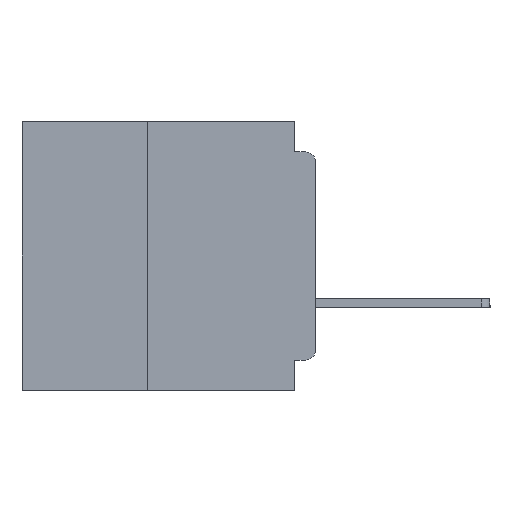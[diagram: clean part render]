
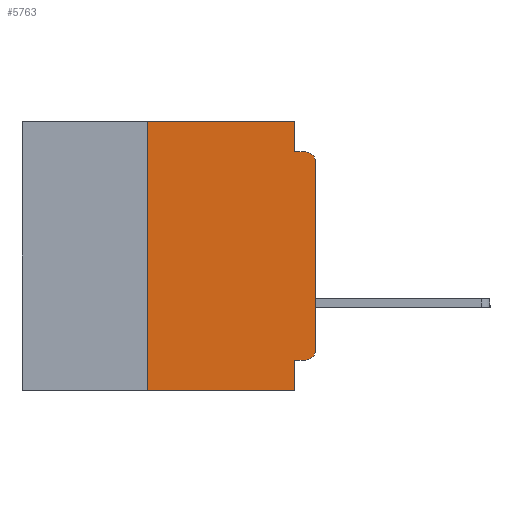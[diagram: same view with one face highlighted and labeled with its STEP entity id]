
A CAD part, left-side view. The second image highlights one B-rep face of the part: STEP entity #5763.
In plain terms, the highlighted planar face has unit normal (-1, 0, 0).
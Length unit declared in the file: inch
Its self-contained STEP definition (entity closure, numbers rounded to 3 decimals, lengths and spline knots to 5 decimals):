
#86 = CARTESIAN_POINT ( 'NONE',  ( 0., 0.437, -0.4 ) ) ;
#521 = EDGE_CURVE ( 'NONE', #8787, #3354, #33060, .T. ) ;
#1106 = ORIENTED_EDGE ( 'NONE', *, *, #25989, .T. ) ;
#1146 = EDGE_LOOP ( 'NONE', ( #22975, #1106, #11759, #16708, #17665, #4040, #8534, #8616, #25637, #13519 ) ) ;
#1576 = CARTESIAN_POINT ( 'NONE',  ( 0., 0.015, -0.06 ) ) ;
#1842 = VERTEX_POINT ( 'NONE', #36062 ) ;
#2887 = VECTOR ( 'NONE', #4983, 39.37008 ) ;
#2947 = CARTESIAN_POINT ( 'NONE',  ( 0., 0.031, 0. ) ) ;
#3354 = VERTEX_POINT ( 'NONE', #25470 ) ;
#3973 = EDGE_CURVE ( 'NONE', #3354, #33789, #15572, .T. ) ;
#4040 = ORIENTED_EDGE ( 'NONE', *, *, #521, .F. ) ;
#4382 = DIRECTION ( 'NONE',  ( 1., 0., 0. ) ) ;
#4648 = DIRECTION ( 'NONE',  ( 0., 0., -1. ) ) ;
#4983 = DIRECTION ( 'NONE',  ( 0., 0., 1. ) ) ;
#5763 = ADVANCED_FACE ( 'NONE', ( #27649 ), #25344, .F. ) ;
#5809 = LINE ( 'NONE', #11395, #28939 ) ;
#6555 = VECTOR ( 'NONE', #24130, 39.37008 ) ;
#7308 = AXIS2_PLACEMENT_3D ( 'NONE', #1576, #22741, #4648 ) ;
#8444 = LINE ( 'NONE', #30062, #6555 ) ;
#8534 = ORIENTED_EDGE ( 'NONE', *, *, #14722, .T. ) ;
#8616 = ORIENTED_EDGE ( 'NONE', *, *, #38856, .F. ) ;
#8787 = VERTEX_POINT ( 'NONE', #9365 ) ;
#9365 = CARTESIAN_POINT ( 'NONE',  ( 0., 0.25, -0.4 ) ) ;
#9541 = DIRECTION ( 'NONE',  ( 0., 0., -1. ) ) ;
#11395 = CARTESIAN_POINT ( 'NONE',  ( 0., 0., -0.045 ) ) ;
#11406 = CARTESIAN_POINT ( 'NONE',  ( 0., 0.015, -0.045 ) ) ;
#11514 = DIRECTION ( 'NONE',  ( 0., -1., 0. ) ) ;
#11759 = ORIENTED_EDGE ( 'NONE', *, *, #18655, .F. ) ;
#12653 = VERTEX_POINT ( 'NONE', #20048 ) ;
#13519 = ORIENTED_EDGE ( 'NONE', *, *, #16425, .T. ) ;
#13583 = DIRECTION ( 'NONE',  ( 0., -1., 0. ) ) ;
#14355 = CARTESIAN_POINT ( 'NONE',  ( 0., 0.031, -0.355 ) ) ;
#14722 = EDGE_CURVE ( 'NONE', #8787, #35647, #21296, .T. ) ;
#15084 = CIRCLE ( 'NONE', #7308, 0.015 ) ;
#15292 = CARTESIAN_POINT ( 'NONE',  ( 0., 0., -0.355 ) ) ;
#15412 = DIRECTION ( 'NONE',  ( 0., 1., 0. ) ) ;
#15527 = DIRECTION ( 'NONE',  ( -1., 0., 0. ) ) ;
#15572 = LINE ( 'NONE', #22582, #22631 ) ;
#15683 = CARTESIAN_POINT ( 'NONE',  ( 0., 0.031, -0.4 ) ) ;
#16425 = EDGE_CURVE ( 'NONE', #1842, #12653, #36123, .T. ) ;
#16708 = ORIENTED_EDGE ( 'NONE', *, *, #31094, .F. ) ;
#17665 = ORIENTED_EDGE ( 'NONE', *, *, #3973, .F. ) ;
#17697 = CARTESIAN_POINT ( 'NONE',  ( 0., 0., -0.06 ) ) ;
#18655 = EDGE_CURVE ( 'NONE', #25463, #28816, #5809, .T. ) ;
#20048 = CARTESIAN_POINT ( 'NONE',  ( 0., 0., -0.34 ) ) ;
#20964 = VECTOR ( 'NONE', #24192, 39.37008 ) ;
#21252 = DIRECTION ( 'NONE',  ( 0., -1., 0. ) ) ;
#21296 = LINE ( 'NONE', #86, #37208 ) ;
#22458 = CARTESIAN_POINT ( 'NONE',  ( 0., 0.437, 0. ) ) ;
#22582 = CARTESIAN_POINT ( 'NONE',  ( 0., 0.437, 0. ) ) ;
#22631 = VECTOR ( 'NONE', #13583, 39.37008 ) ;
#22741 = DIRECTION ( 'NONE',  ( -1., 0., 0. ) ) ;
#22803 = VERTEX_POINT ( 'NONE', #14355 ) ;
#22975 = ORIENTED_EDGE ( 'NONE', *, *, #28309, .T. ) ;
#23720 = AXIS2_PLACEMENT_3D ( 'NONE', #22458, #4382, #25475 ) ;
#24130 = DIRECTION ( 'NONE',  ( 0., 0., 1. ) ) ;
#24192 = DIRECTION ( 'NONE',  ( 0., 0., -1. ) ) ;
#25344 = PLANE ( 'NONE',  #23720 ) ;
#25463 = VERTEX_POINT ( 'NONE', #38220 ) ;
#25470 = CARTESIAN_POINT ( 'NONE',  ( 0., 0.25, 0. ) ) ;
#25475 = DIRECTION ( 'NONE',  ( 0., 0., -1. ) ) ;
#25637 = ORIENTED_EDGE ( 'NONE', *, *, #33869, .F. ) ;
#25989 = EDGE_CURVE ( 'NONE', #36343, #28816, #15084, .T. ) ;
#26809 = CARTESIAN_POINT ( 'NONE',  ( 0., 0.25, -0.4 ) ) ;
#27649 = FACE_OUTER_BOUND ( 'NONE', #1146, .T. ) ;
#28309 = EDGE_CURVE ( 'NONE', #12653, #36343, #8444, .T. ) ;
#28816 = VERTEX_POINT ( 'NONE', #11406 ) ;
#28939 = VECTOR ( 'NONE', #11514, 39.37008 ) ;
#28982 = LINE ( 'NONE', #2947, #20964 ) ;
#29943 = VECTOR ( 'NONE', #15412, 39.37008 ) ;
#30062 = CARTESIAN_POINT ( 'NONE',  ( 0., 0., 0. ) ) ;
#31094 = EDGE_CURVE ( 'NONE', #33789, #25463, #28982, .T. ) ;
#32571 = CARTESIAN_POINT ( 'NONE',  ( 0., 0.031, -0.4 ) ) ;
#33060 = LINE ( 'NONE', #26809, #2887 ) ;
#33516 = CARTESIAN_POINT ( 'NONE',  ( 0., 0.015, -0.34 ) ) ;
#33789 = VERTEX_POINT ( 'NONE', #38746 ) ;
#33869 = EDGE_CURVE ( 'NONE', #1842, #22803, #38789, .T. ) ;
#35641 = VECTOR ( 'NONE', #9541, 39.37008 ) ;
#35647 = VERTEX_POINT ( 'NONE', #32571 ) ;
#36062 = CARTESIAN_POINT ( 'NONE',  ( 0., 0.015, -0.355 ) ) ;
#36123 = CIRCLE ( 'NONE', #36284, 0.015 ) ;
#36284 = AXIS2_PLACEMENT_3D ( 'NONE', #33516, #15527, #36528 ) ;
#36343 = VERTEX_POINT ( 'NONE', #17697 ) ;
#36528 = DIRECTION ( 'NONE',  ( 0., 0., -1. ) ) ;
#36582 = LINE ( 'NONE', #15683, #35641 ) ;
#37208 = VECTOR ( 'NONE', #21252, 39.37008 ) ;
#38220 = CARTESIAN_POINT ( 'NONE',  ( 0., 0.031, -0.045 ) ) ;
#38746 = CARTESIAN_POINT ( 'NONE',  ( 0., 0.031, 0. ) ) ;
#38789 = LINE ( 'NONE', #15292, #29943 ) ;
#38856 = EDGE_CURVE ( 'NONE', #22803, #35647, #36582, .T. ) ;
